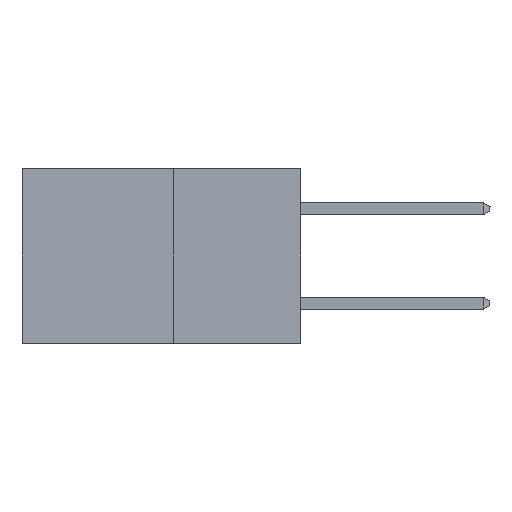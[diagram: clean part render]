
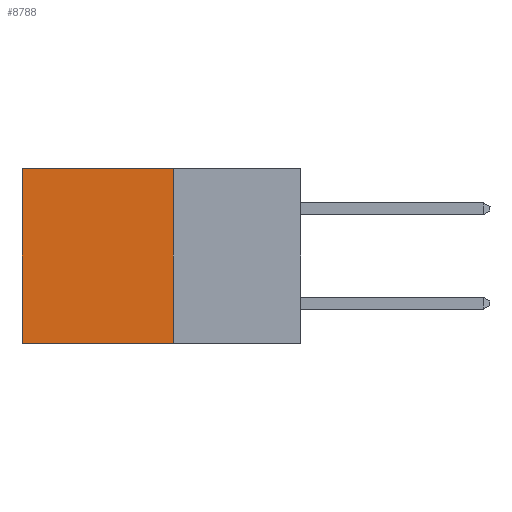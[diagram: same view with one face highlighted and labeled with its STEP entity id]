
A CAD part, left-side view. The second image highlights one B-rep face of the part: STEP entity #8788.
In plain terms, the highlighted planar face has unit normal (-1, 0, 0).
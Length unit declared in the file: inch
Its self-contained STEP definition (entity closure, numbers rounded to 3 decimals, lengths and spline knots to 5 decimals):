
#312 = CARTESIAN_POINT ( 'NONE',  ( 0.277, 0.27, -0.37 ) ) ;
#595 = DIRECTION ( 'NONE',  ( 0., 0., -1. ) ) ;
#1252 = FACE_OUTER_BOUND ( 'NONE', #3816, .T. ) ;
#1484 = VECTOR ( 'NONE', #3517, 39.37008 ) ;
#1666 = AXIS2_PLACEMENT_3D ( 'NONE', #7882, #4040, #9349 ) ;
#1792 = CARTESIAN_POINT ( 'NONE',  ( 0.277, 0.27, 0. ) ) ;
#2185 = EDGE_CURVE ( 'NONE', #7568, #3453, #4059, .T. ) ;
#2365 = PLANE ( 'NONE',  #1666 ) ;
#2720 = EDGE_CURVE ( 'NONE', #4985, #4379, #9145, .T. ) ;
#2749 = DIRECTION ( 'NONE',  ( 0., 1., 0. ) ) ;
#3279 = VECTOR ( 'NONE', #2749, 39.37008 ) ;
#3301 = CARTESIAN_POINT ( 'NONE',  ( 0.277, 0.27, -0.37 ) ) ;
#3453 = VERTEX_POINT ( 'NONE', #8963 ) ;
#3517 = DIRECTION ( 'NONE',  ( 0., 0., -1. ) ) ;
#3816 = EDGE_LOOP ( 'NONE', ( #5736, #8414, #9341, #7861 ) ) ;
#4040 = DIRECTION ( 'NONE',  ( 1., 0., 0. ) ) ;
#4059 = LINE ( 'NONE', #8911, #3279 ) ;
#4379 = VERTEX_POINT ( 'NONE', #6988 ) ;
#4434 = DIRECTION ( 'NONE',  ( 0., 1., 0. ) ) ;
#4985 = VERTEX_POINT ( 'NONE', #312 ) ;
#5736 = ORIENTED_EDGE ( 'NONE', *, *, #9256, .T. ) ;
#6645 = VECTOR ( 'NONE', #595, 39.37008 ) ;
#6988 = CARTESIAN_POINT ( 'NONE',  ( 0.277, 0.59, -0.37 ) ) ;
#7224 = VECTOR ( 'NONE', #4434, 39.37008 ) ;
#7446 = CARTESIAN_POINT ( 'NONE',  ( 0.277, 0.27, -0.37 ) ) ;
#7568 = VERTEX_POINT ( 'NONE', #1792 ) ;
#7861 = ORIENTED_EDGE ( 'NONE', *, *, #2185, .T. ) ;
#7882 = CARTESIAN_POINT ( 'NONE',  ( 0.277, 0.27, -0.37 ) ) ;
#8414 = ORIENTED_EDGE ( 'NONE', *, *, #2720, .F. ) ;
#8788 = ADVANCED_FACE ( 'NONE', ( #1252 ), #2365, .F. ) ;
#8849 = LINE ( 'NONE', #9930, #6645 ) ;
#8911 = CARTESIAN_POINT ( 'NONE',  ( 0.277, 0.27, 0. ) ) ;
#8963 = CARTESIAN_POINT ( 'NONE',  ( 0.277, 0.59, 0. ) ) ;
#9145 = LINE ( 'NONE', #3301, #7224 ) ;
#9256 = EDGE_CURVE ( 'NONE', #3453, #4379, #8849, .T. ) ;
#9341 = ORIENTED_EDGE ( 'NONE', *, *, #9624, .F. ) ;
#9349 = DIRECTION ( 'NONE',  ( 0., 0., -1. ) ) ;
#9518 = LINE ( 'NONE', #7446, #1484 ) ;
#9624 = EDGE_CURVE ( 'NONE', #7568, #4985, #9518, .T. ) ;
#9930 = CARTESIAN_POINT ( 'NONE',  ( 0.277, 0.59, -0.37 ) ) ;
